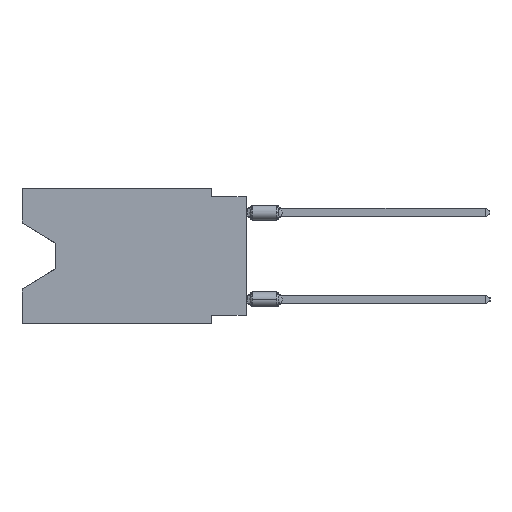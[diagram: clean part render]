
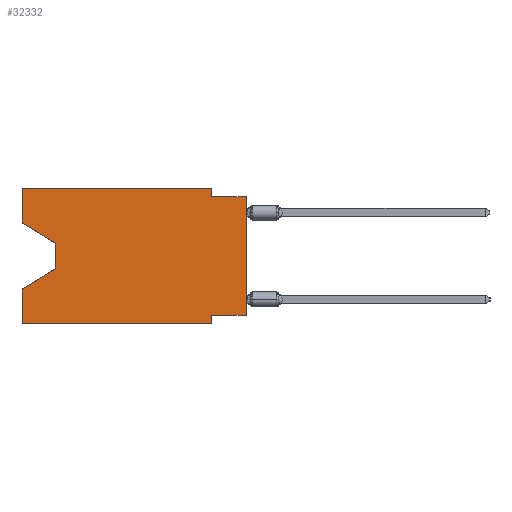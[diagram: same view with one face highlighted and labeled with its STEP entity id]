
A CAD part, left-side view. The second image highlights one B-rep face of the part: STEP entity #32332.
In plain terms, the highlighted planar face has unit normal (-1, 0, 0).
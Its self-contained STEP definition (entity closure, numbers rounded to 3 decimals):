
#642 = ORIENTED_EDGE ( 'NONE', *, *, #58067, .T. ) ;
#1279 = LINE ( 'NONE', #42907, #2857 ) ;
#1645 = VECTOR ( 'NONE', #17136, 1000. ) ;
#1739 = LINE ( 'NONE', #20011, #13583 ) ;
#2857 = VECTOR ( 'NONE', #56104, 1000. ) ;
#3822 = CARTESIAN_POINT ( 'NONE',  ( 0., 13.97, -5.893 ) ) ;
#5438 = CARTESIAN_POINT ( 'NONE',  ( 0., 2.54, -0.635 ) ) ;
#6791 = CARTESIAN_POINT ( 'NONE',  ( 0., 16.383, 0. ) ) ;
#6994 = ORIENTED_EDGE ( 'NONE', *, *, #48582, .F. ) ;
#7083 = LINE ( 'NONE', #6791, #38093 ) ;
#7245 = CARTESIAN_POINT ( 'NONE',  ( 0., 0., 0. ) ) ;
#8994 = EDGE_CURVE ( 'NONE', #32551, #25263, #12209, .T. ) ;
#9034 = ORIENTED_EDGE ( 'NONE', *, *, #34672, .F. ) ;
#10389 = LINE ( 'NONE', #19679, #27882 ) ;
#11612 = EDGE_CURVE ( 'NONE', #53486, #12280, #40908, .T. ) ;
#12042 = DIRECTION ( 'NONE',  ( 0., 0., -1. ) ) ;
#12159 = ORIENTED_EDGE ( 'NONE', *, *, #12332, .F. ) ;
#12209 = LINE ( 'NONE', #3822, #17282 ) ;
#12280 = VERTEX_POINT ( 'NONE', #40120 ) ;
#12332 = EDGE_CURVE ( 'NONE', #29221, #24620, #26941, .T. ) ;
#12574 = EDGE_CURVE ( 'NONE', #56821, #15135, #1739, .T. ) ;
#12942 = LINE ( 'NONE', #25521, #33064 ) ;
#13224 = DIRECTION ( 'NONE',  ( 0., 0., -1. ) ) ;
#13460 = DIRECTION ( 'NONE',  ( 0., 0., 1. ) ) ;
#13583 = VECTOR ( 'NONE', #56575, 1000. ) ;
#13678 = VECTOR ( 'NONE', #40330, 1000. ) ;
#14818 = CARTESIAN_POINT ( 'NONE',  ( 0., 2.54, -9.271 ) ) ;
#15135 = VERTEX_POINT ( 'NONE', #14818 ) ;
#16838 = CARTESIAN_POINT ( 'NONE',  ( 0., 16.383, -2.546 ) ) ;
#17136 = DIRECTION ( 'NONE',  ( 0., 0., 1. ) ) ;
#17282 = VECTOR ( 'NONE', #44263, 1000. ) ;
#19050 = CARTESIAN_POINT ( 'NONE',  ( 0., 13.97, -5.893 ) ) ;
#19335 = EDGE_CURVE ( 'NONE', #29221, #59033, #10389, .T. ) ;
#19366 = VECTOR ( 'NONE', #13460, 1000. ) ;
#19679 = CARTESIAN_POINT ( 'NONE',  ( 0., 16.383, -2.546 ) ) ;
#20011 = CARTESIAN_POINT ( 'NONE',  ( 0., 0., -9.271 ) ) ;
#20078 = DIRECTION ( 'NONE',  ( 1., 0., 0. ) ) ;
#20282 = DIRECTION ( 'NONE',  ( 0., 0., -1. ) ) ;
#21117 = VECTOR ( 'NONE', #13224, 1000. ) ;
#21349 = ORIENTED_EDGE ( 'NONE', *, *, #31896, .T. ) ;
#21358 = EDGE_CURVE ( 'NONE', #24620, #48081, #55792, .T. ) ;
#22444 = CARTESIAN_POINT ( 'NONE',  ( 0., 16.383, 0. ) ) ;
#22501 = CARTESIAN_POINT ( 'NONE',  ( 0., 2.54, 0. ) ) ;
#23979 = PLANE ( 'NONE',  #29259 ) ;
#24389 = VERTEX_POINT ( 'NONE', #40739 ) ;
#24620 = VERTEX_POINT ( 'NONE', #51813 ) ;
#25263 = VERTEX_POINT ( 'NONE', #48416 ) ;
#25348 = DIRECTION ( 'NONE',  ( 0., 0., 1. ) ) ;
#25477 = ORIENTED_EDGE ( 'NONE', *, *, #31954, .T. ) ;
#25521 = CARTESIAN_POINT ( 'NONE',  ( 0., 13.97, -4.013 ) ) ;
#26576 = DIRECTION ( 'NONE',  ( 0., 0., -1. ) ) ;
#26828 = VERTEX_POINT ( 'NONE', #58402 ) ;
#26941 = LINE ( 'NONE', #22444, #19366 ) ;
#27882 = VECTOR ( 'NONE', #47240, 1000. ) ;
#29221 = VERTEX_POINT ( 'NONE', #16838 ) ;
#29259 = AXIS2_PLACEMENT_3D ( 'NONE', #47045, #20078, #26576 ) ;
#31896 = EDGE_CURVE ( 'NONE', #56821, #12280, #53387, .T. ) ;
#31954 = EDGE_CURVE ( 'NONE', #59033, #32551, #12942, .T. ) ;
#32332 = ADVANCED_FACE ( 'NONE', ( #32951 ), #23979, .F. ) ;
#32551 = VERTEX_POINT ( 'NONE', #19050 ) ;
#32951 = FACE_OUTER_BOUND ( 'NONE', #42639, .T. ) ;
#33064 = VECTOR ( 'NONE', #12042, 1000. ) ;
#33300 = DIRECTION ( 'NONE',  ( 0., -1., 0. ) ) ;
#34343 = LINE ( 'NONE', #57136, #40183 ) ;
#34672 = EDGE_CURVE ( 'NONE', #26828, #25263, #7083, .T. ) ;
#35036 = ORIENTED_EDGE ( 'NONE', *, *, #21358, .F. ) ;
#35924 = ORIENTED_EDGE ( 'NONE', *, *, #49516, .F. ) ;
#38013 = CARTESIAN_POINT ( 'NONE',  ( 0., 2.54, 0. ) ) ;
#38093 = VECTOR ( 'NONE', #25348, 1000. ) ;
#38910 = CARTESIAN_POINT ( 'NONE',  ( 0., 0., -9.271 ) ) ;
#40120 = CARTESIAN_POINT ( 'NONE',  ( 0., 0., -0.635 ) ) ;
#40183 = VECTOR ( 'NONE', #20282, 1000. ) ;
#40330 = DIRECTION ( 'NONE',  ( 0., -1., 0. ) ) ;
#40739 = CARTESIAN_POINT ( 'NONE',  ( 0., 2.54, -9.906 ) ) ;
#40908 = LINE ( 'NONE', #59217, #13678 ) ;
#42381 = VECTOR ( 'NONE', #33300, 1000. ) ;
#42594 = CARTESIAN_POINT ( 'NONE',  ( 0., 16.383, 0. ) ) ;
#42639 = EDGE_LOOP ( 'NONE', ( #50746, #25477, #52593, #9034, #642, #6994, #46623, #21349, #46460, #35924, #35036, #12159 ) ) ;
#42907 = CARTESIAN_POINT ( 'NONE',  ( 0., 16.383, -9.906 ) ) ;
#44263 = DIRECTION ( 'NONE',  ( 0., 0.855, -0.519 ) ) ;
#46460 = ORIENTED_EDGE ( 'NONE', *, *, #11612, .F. ) ;
#46623 = ORIENTED_EDGE ( 'NONE', *, *, #12574, .F. ) ;
#47045 = CARTESIAN_POINT ( 'NONE',  ( 0., 16.383, 0. ) ) ;
#47240 = DIRECTION ( 'NONE',  ( 0., -0.855, -0.519 ) ) ;
#48081 = VERTEX_POINT ( 'NONE', #38013 ) ;
#48416 = CARTESIAN_POINT ( 'NONE',  ( 0., 16.383, -7.36 ) ) ;
#48582 = EDGE_CURVE ( 'NONE', #15135, #24389, #34343, .T. ) ;
#49516 = EDGE_CURVE ( 'NONE', #48081, #53486, #58777, .T. ) ;
#50746 = ORIENTED_EDGE ( 'NONE', *, *, #19335, .T. ) ;
#51813 = CARTESIAN_POINT ( 'NONE',  ( 0., 16.383, 0. ) ) ;
#52593 = ORIENTED_EDGE ( 'NONE', *, *, #8994, .T. ) ;
#53387 = LINE ( 'NONE', #7245, #1645 ) ;
#53486 = VERTEX_POINT ( 'NONE', #5438 ) ;
#54175 = CARTESIAN_POINT ( 'NONE',  ( 0., 13.97, -4.013 ) ) ;
#55792 = LINE ( 'NONE', #42594, #42381 ) ;
#56104 = DIRECTION ( 'NONE',  ( 0., -1., 0. ) ) ;
#56575 = DIRECTION ( 'NONE',  ( 0., 1., 0. ) ) ;
#56821 = VERTEX_POINT ( 'NONE', #38910 ) ;
#57136 = CARTESIAN_POINT ( 'NONE',  ( 0., 2.54, -9.906 ) ) ;
#58067 = EDGE_CURVE ( 'NONE', #26828, #24389, #1279, .T. ) ;
#58402 = CARTESIAN_POINT ( 'NONE',  ( 0., 16.383, -9.906 ) ) ;
#58777 = LINE ( 'NONE', #22501, #21117 ) ;
#59033 = VERTEX_POINT ( 'NONE', #54175 ) ;
#59217 = CARTESIAN_POINT ( 'NONE',  ( 0., 0., -0.635 ) ) ;
